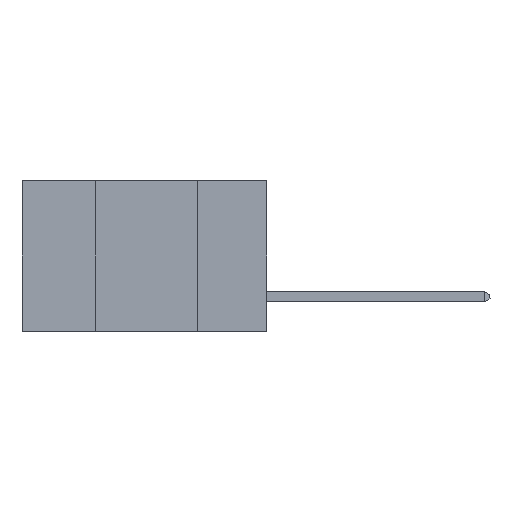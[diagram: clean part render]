
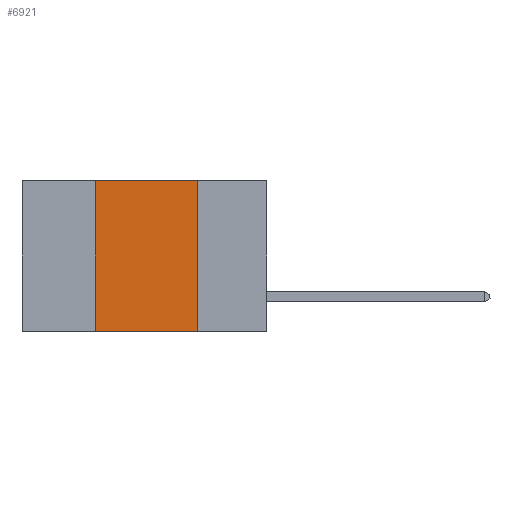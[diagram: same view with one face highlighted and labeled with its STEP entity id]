
A CAD part, left-side view. The second image highlights one B-rep face of the part: STEP entity #6921.
In plain terms, the highlighted planar face has unit normal (-1, 0, 0).
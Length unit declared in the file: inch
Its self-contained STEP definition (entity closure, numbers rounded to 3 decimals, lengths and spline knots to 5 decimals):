
#114 = EDGE_CURVE ( 'NONE', #1513, #4103, #8490, .T. ) ;
#176 = LINE ( 'NONE', #4051, #6296 ) ;
#294 = EDGE_CURVE ( 'NONE', #8282, #7884, #176, .T. ) ;
#454 = EDGE_CURVE ( 'NONE', #8282, #1513, #4311, .T. ) ;
#658 = ORIENTED_EDGE ( 'NONE', *, *, #8440, .F. ) ;
#1118 = EDGE_LOOP ( 'NONE', ( #658, #5189, #6922, #2900 ) ) ;
#1466 = CARTESIAN_POINT ( 'NONE',  ( 0., 0.42, 0. ) ) ;
#1513 = VERTEX_POINT ( 'NONE', #2361 ) ;
#2361 = CARTESIAN_POINT ( 'NONE',  ( 0., 0.42, 0. ) ) ;
#2900 = ORIENTED_EDGE ( 'NONE', *, *, #294, .T. ) ;
#3043 = VECTOR ( 'NONE', #8100, 39.37008 ) ;
#3166 = CARTESIAN_POINT ( 'NONE',  ( 0., 0.42, -0.37 ) ) ;
#3324 = DIRECTION ( 'NONE',  ( 0., 0., -1. ) ) ;
#3354 = CARTESIAN_POINT ( 'NONE',  ( 0., 0.17, 0. ) ) ;
#3843 = DIRECTION ( 'NONE',  ( 1., 0., 0. ) ) ;
#4051 = CARTESIAN_POINT ( 'NONE',  ( 0., 0.6, -0.37 ) ) ;
#4103 = VERTEX_POINT ( 'NONE', #8957 ) ;
#4111 = DIRECTION ( 'NONE',  ( 0., -1., 0. ) ) ;
#4311 = LINE ( 'NONE', #1466, #3043 ) ;
#4723 = CARTESIAN_POINT ( 'NONE',  ( 0., 0.17, -0.37 ) ) ;
#5148 = VECTOR ( 'NONE', #7243, 39.37008 ) ;
#5189 = ORIENTED_EDGE ( 'NONE', *, *, #114, .F. ) ;
#6043 = CARTESIAN_POINT ( 'NONE',  ( 0., 0.6, 0. ) ) ;
#6296 = VECTOR ( 'NONE', #4111, 39.37008 ) ;
#6643 = LINE ( 'NONE', #3354, #7887 ) ;
#6868 = DIRECTION ( 'NONE',  ( 0., 0., -1. ) ) ;
#6921 = ADVANCED_FACE ( 'NONE', ( #8152 ), #7644, .F. ) ;
#6922 = ORIENTED_EDGE ( 'NONE', *, *, #454, .F. ) ;
#7243 = DIRECTION ( 'NONE',  ( 0., -1., 0. ) ) ;
#7644 = PLANE ( 'NONE',  #8748 ) ;
#7884 = VERTEX_POINT ( 'NONE', #4723 ) ;
#7887 = VECTOR ( 'NONE', #3324, 39.37008 ) ;
#8100 = DIRECTION ( 'NONE',  ( 0., 0., 1. ) ) ;
#8152 = FACE_OUTER_BOUND ( 'NONE', #1118, .T. ) ;
#8282 = VERTEX_POINT ( 'NONE', #3166 ) ;
#8440 = EDGE_CURVE ( 'NONE', #4103, #7884, #6643, .T. ) ;
#8490 = LINE ( 'NONE', #9529, #5148 ) ;
#8748 = AXIS2_PLACEMENT_3D ( 'NONE', #6043, #3843, #6868 ) ;
#8957 = CARTESIAN_POINT ( 'NONE',  ( 0., 0.17, 0. ) ) ;
#9529 = CARTESIAN_POINT ( 'NONE',  ( 0., 0.6, 0. ) ) ;
